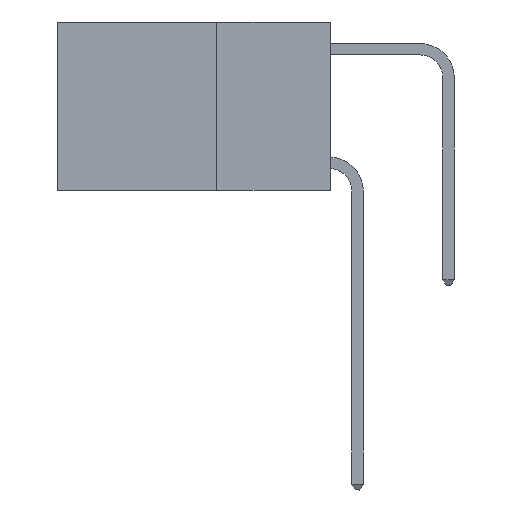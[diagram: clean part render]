
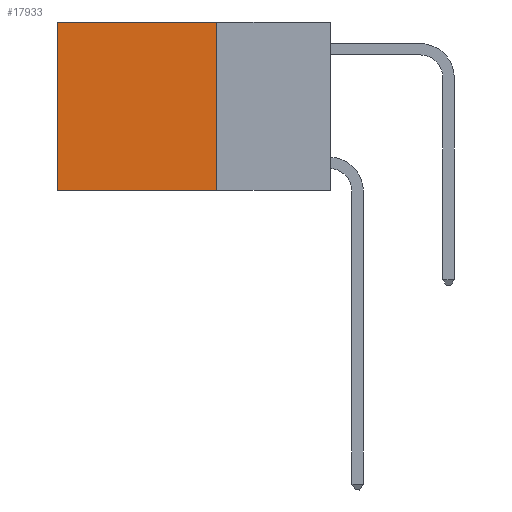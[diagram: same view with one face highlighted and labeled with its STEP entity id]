
A CAD part, left-side view. The second image highlights one B-rep face of the part: STEP entity #17933.
In plain terms, the highlighted planar face has unit normal (-1, 0, 0).
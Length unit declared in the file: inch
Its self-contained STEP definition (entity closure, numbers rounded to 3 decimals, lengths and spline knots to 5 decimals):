
#211 = LINE ( 'NONE', #12422, #7970 ) ;
#261 = VERTEX_POINT ( 'NONE', #14088 ) ;
#1464 = CARTESIAN_POINT ( 'NONE',  ( 0.2625, 0.25, 0. ) ) ;
#1547 = ORIENTED_EDGE ( 'NONE', *, *, #8423, .T. ) ;
#1799 = ORIENTED_EDGE ( 'NONE', *, *, #6030, .F. ) ;
#1868 = ORIENTED_EDGE ( 'NONE', *, *, #6729, .T. ) ;
#3065 = DIRECTION ( 'NONE',  ( 0., 0., -1. ) ) ;
#3105 = CARTESIAN_POINT ( 'NONE',  ( 0.2625, 0.25, 0. ) ) ;
#3297 = VERTEX_POINT ( 'NONE', #14427 ) ;
#3520 = VECTOR ( 'NONE', #5529, 39.37008 ) ;
#4927 = DIRECTION ( 'NONE',  ( 0., 1., 0. ) ) ;
#5529 = DIRECTION ( 'NONE',  ( 0., 0., -1. ) ) ;
#6030 = EDGE_CURVE ( 'NONE', #17651, #3297, #18023, .T. ) ;
#6214 = VECTOR ( 'NONE', #3065, 39.37008 ) ;
#6615 = CARTESIAN_POINT ( 'NONE',  ( 0.2625, 0.25, 0. ) ) ;
#6729 = EDGE_CURVE ( 'NONE', #17651, #261, #14377, .T. ) ;
#7601 = LINE ( 'NONE', #13000, #3520 ) ;
#7970 = VECTOR ( 'NONE', #4927, 39.37008 ) ;
#8027 = VERTEX_POINT ( 'NONE', #9125 ) ;
#8121 = DIRECTION ( 'NONE',  ( 0., 0., -1. ) ) ;
#8354 = ORIENTED_EDGE ( 'NONE', *, *, #11424, .F. ) ;
#8423 = EDGE_CURVE ( 'NONE', #261, #8027, #7601, .T. ) ;
#9125 = CARTESIAN_POINT ( 'NONE',  ( 0.2625, 0.6, -0.37 ) ) ;
#9249 = DIRECTION ( 'NONE',  ( 0., 1., 0. ) ) ;
#9485 = EDGE_LOOP ( 'NONE', ( #1547, #8354, #1799, #1868 ) ) ;
#9497 = AXIS2_PLACEMENT_3D ( 'NONE', #6615, #17002, #8121 ) ;
#11424 = EDGE_CURVE ( 'NONE', #3297, #8027, #211, .T. ) ;
#12422 = CARTESIAN_POINT ( 'NONE',  ( 0.2625, 0.25, -0.37 ) ) ;
#13000 = CARTESIAN_POINT ( 'NONE',  ( 0.2625, 0.6, 0. ) ) ;
#13516 = FACE_OUTER_BOUND ( 'NONE', #9485, .T. ) ;
#14088 = CARTESIAN_POINT ( 'NONE',  ( 0.2625, 0.6, 0. ) ) ;
#14377 = LINE ( 'NONE', #3105, #19060 ) ;
#14427 = CARTESIAN_POINT ( 'NONE',  ( 0.2625, 0.25, -0.37 ) ) ;
#14587 = CARTESIAN_POINT ( 'NONE',  ( 0.2625, 0.25, 0. ) ) ;
#17002 = DIRECTION ( 'NONE',  ( 1., 0., 0. ) ) ;
#17651 = VERTEX_POINT ( 'NONE', #14587 ) ;
#17933 = ADVANCED_FACE ( 'NONE', ( #13516 ), #18350, .F. ) ;
#18023 = LINE ( 'NONE', #1464, #6214 ) ;
#18350 = PLANE ( 'NONE',  #9497 ) ;
#19060 = VECTOR ( 'NONE', #9249, 39.37008 ) ;
